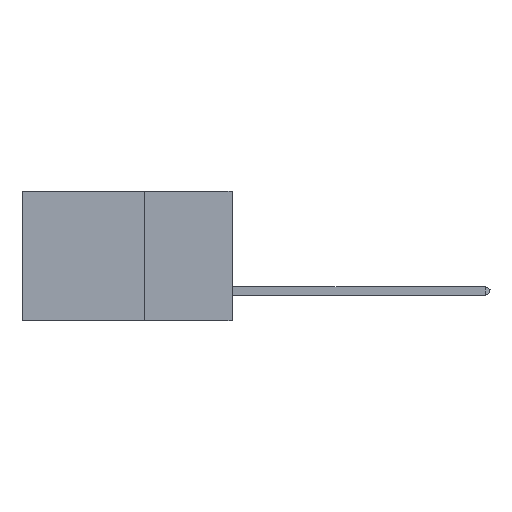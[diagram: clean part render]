
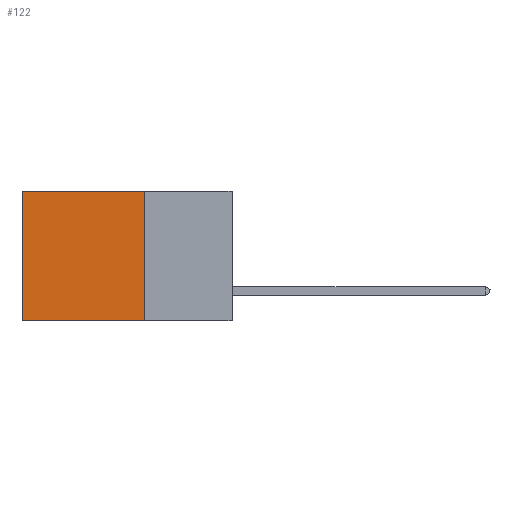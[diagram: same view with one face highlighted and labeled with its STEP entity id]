
A CAD part, left-side view. The second image highlights one B-rep face of the part: STEP entity #122.
In plain terms, the highlighted planar face has unit normal (-1, 0, 0).
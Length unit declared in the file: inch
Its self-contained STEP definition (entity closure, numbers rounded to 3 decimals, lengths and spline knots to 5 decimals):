
#122 = ADVANCED_FACE ( 'NONE', ( #9688 ), #26222, .F. ) ;
#871 = CARTESIAN_POINT ( 'NONE',  ( 0.2875, 0.25, 0. ) ) ;
#2534 = CARTESIAN_POINT ( 'NONE',  ( 0.2875, 0.6, 0. ) ) ;
#2710 = VERTEX_POINT ( 'NONE', #2534 ) ;
#2792 = VECTOR ( 'NONE', #39859, 39.37008 ) ;
#3507 = CARTESIAN_POINT ( 'NONE',  ( 0.2875, 0.25, 0. ) ) ;
#5293 = EDGE_CURVE ( 'NONE', #34335, #14742, #30658, .T. ) ;
#5485 = LINE ( 'NONE', #3507, #35689 ) ;
#5881 = VERTEX_POINT ( 'NONE', #42019 ) ;
#6679 = ORIENTED_EDGE ( 'NONE', *, *, #18762, .F. ) ;
#6741 = DIRECTION ( 'NONE',  ( 1., 0., 0. ) ) ;
#6878 = CARTESIAN_POINT ( 'NONE',  ( 0.2875, 0.6, -0.37 ) ) ;
#9688 = FACE_OUTER_BOUND ( 'NONE', #39630, .T. ) ;
#10680 = ORIENTED_EDGE ( 'NONE', *, *, #27953, .T. ) ;
#14742 = VERTEX_POINT ( 'NONE', #6878 ) ;
#18762 = EDGE_CURVE ( 'NONE', #5881, #34335, #5485, .T. ) ;
#19483 = EDGE_CURVE ( 'NONE', #2710, #14742, #49615, .T. ) ;
#21019 = DIRECTION ( 'NONE',  ( 0., 0., -1. ) ) ;
#23449 = ORIENTED_EDGE ( 'NONE', *, *, #19483, .T. ) ;
#23697 = VECTOR ( 'NONE', #39900, 39.37008 ) ;
#26222 = PLANE ( 'NONE',  #34415 ) ;
#27316 = CARTESIAN_POINT ( 'NONE',  ( 0.2875, 0.25, -0.37 ) ) ;
#27953 = EDGE_CURVE ( 'NONE', #5881, #2710, #47030, .T. ) ;
#30116 = DIRECTION ( 'NONE',  ( 0., 0., -1. ) ) ;
#30658 = LINE ( 'NONE', #36014, #2792 ) ;
#32732 = VECTOR ( 'NONE', #21019, 39.37008 ) ;
#34269 = CARTESIAN_POINT ( 'NONE',  ( 0.2875, 0.25, 0. ) ) ;
#34335 = VERTEX_POINT ( 'NONE', #27316 ) ;
#34415 = AXIS2_PLACEMENT_3D ( 'NONE', #34269, #6741, #30116 ) ;
#35689 = VECTOR ( 'NONE', #45075, 39.37008 ) ;
#36014 = CARTESIAN_POINT ( 'NONE',  ( 0.2875, 0.25, -0.37 ) ) ;
#39630 = EDGE_LOOP ( 'NONE', ( #23449, #46470, #6679, #10680 ) ) ;
#39662 = CARTESIAN_POINT ( 'NONE',  ( 0.2875, 0.6, 0. ) ) ;
#39859 = DIRECTION ( 'NONE',  ( 0., 1., 0. ) ) ;
#39900 = DIRECTION ( 'NONE',  ( 0., 1., 0. ) ) ;
#42019 = CARTESIAN_POINT ( 'NONE',  ( 0.2875, 0.25, 0. ) ) ;
#45075 = DIRECTION ( 'NONE',  ( 0., 0., -1. ) ) ;
#46470 = ORIENTED_EDGE ( 'NONE', *, *, #5293, .F. ) ;
#47030 = LINE ( 'NONE', #871, #23697 ) ;
#49615 = LINE ( 'NONE', #39662, #32732 ) ;
